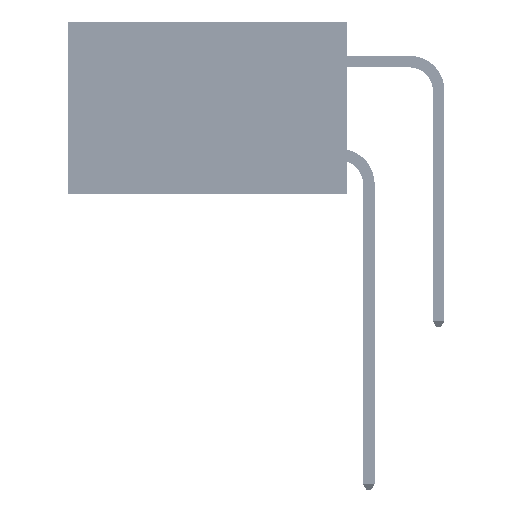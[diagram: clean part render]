
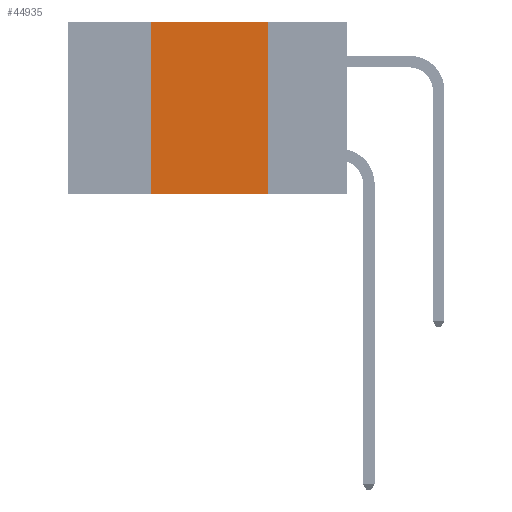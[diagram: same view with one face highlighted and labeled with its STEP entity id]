
A CAD part, left-side view. The second image highlights one B-rep face of the part: STEP entity #44935.
In plain terms, the highlighted planar face has unit normal (-1, 0, 0).
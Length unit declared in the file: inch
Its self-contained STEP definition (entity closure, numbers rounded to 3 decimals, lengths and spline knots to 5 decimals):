
#772 = CARTESIAN_POINT ( 'NONE',  ( 0., 0.6, -0.37 ) ) ;
#1287 = VECTOR ( 'NONE', #25290, 39.37008 ) ;
#1383 = CARTESIAN_POINT ( 'NONE',  ( 0., 0.17, 0. ) ) ;
#1932 = EDGE_CURVE ( 'NONE', #46234, #12027, #24584, .T. ) ;
#2560 = CARTESIAN_POINT ( 'NONE',  ( 0., 0.42, -0.37 ) ) ;
#2838 = VECTOR ( 'NONE', #40467, 39.37008 ) ;
#3495 = AXIS2_PLACEMENT_3D ( 'NONE', #24012, #5701, #16789 ) ;
#3510 = ORIENTED_EDGE ( 'NONE', *, *, #33971, .T. ) ;
#4608 = ORIENTED_EDGE ( 'NONE', *, *, #14928, .F. ) ;
#5701 = DIRECTION ( 'NONE',  ( 1., 0., 0. ) ) ;
#8233 = DIRECTION ( 'NONE',  ( 0., -1., 0. ) ) ;
#8610 = EDGE_CURVE ( 'NONE', #23495, #12387, #22201, .T. ) ;
#9328 = FACE_OUTER_BOUND ( 'NONE', #16380, .T. ) ;
#10676 = DIRECTION ( 'NONE',  ( 0., -1., 0. ) ) ;
#10771 = ORIENTED_EDGE ( 'NONE', *, *, #1932, .F. ) ;
#11366 = CARTESIAN_POINT ( 'NONE',  ( 0., 0.17, 0. ) ) ;
#12027 = VERTEX_POINT ( 'NONE', #13487 ) ;
#12387 = VERTEX_POINT ( 'NONE', #23788 ) ;
#13487 = CARTESIAN_POINT ( 'NONE',  ( 0., 0.42, 0. ) ) ;
#14270 = LINE ( 'NONE', #21509, #15345 ) ;
#14928 = EDGE_CURVE ( 'NONE', #12027, #23495, #14270, .T. ) ;
#15345 = VECTOR ( 'NONE', #10676, 39.37008 ) ;
#16380 = EDGE_LOOP ( 'NONE', ( #36651, #4608, #10771, #3510 ) ) ;
#16789 = DIRECTION ( 'NONE',  ( 0., 0., -1. ) ) ;
#21509 = CARTESIAN_POINT ( 'NONE',  ( 0., 0.6, 0. ) ) ;
#22201 = LINE ( 'NONE', #11366, #2838 ) ;
#23495 = VERTEX_POINT ( 'NONE', #1383 ) ;
#23788 = CARTESIAN_POINT ( 'NONE',  ( 0., 0.17, -0.37 ) ) ;
#24012 = CARTESIAN_POINT ( 'NONE',  ( 0., 0.6, 0. ) ) ;
#24584 = LINE ( 'NONE', #32512, #1287 ) ;
#25290 = DIRECTION ( 'NONE',  ( 0., 0., 1. ) ) ;
#32512 = CARTESIAN_POINT ( 'NONE',  ( 0., 0.42, 0. ) ) ;
#33971 = EDGE_CURVE ( 'NONE', #46234, #12387, #34463, .T. ) ;
#34463 = LINE ( 'NONE', #772, #47212 ) ;
#35320 = PLANE ( 'NONE',  #3495 ) ;
#36651 = ORIENTED_EDGE ( 'NONE', *, *, #8610, .F. ) ;
#40467 = DIRECTION ( 'NONE',  ( 0., 0., -1. ) ) ;
#44935 = ADVANCED_FACE ( 'NONE', ( #9328 ), #35320, .F. ) ;
#46234 = VERTEX_POINT ( 'NONE', #2560 ) ;
#47212 = VECTOR ( 'NONE', #8233, 39.37008 ) ;
